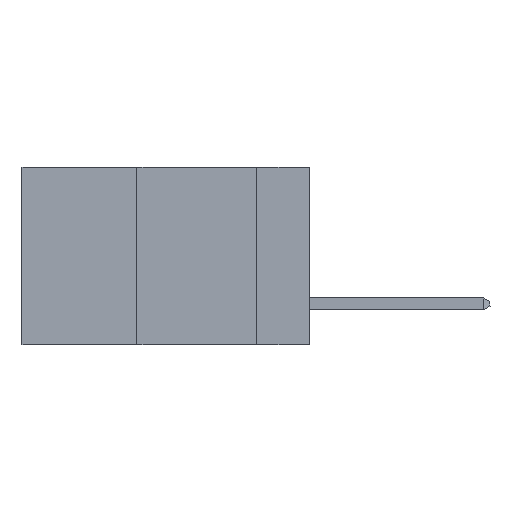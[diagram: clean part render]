
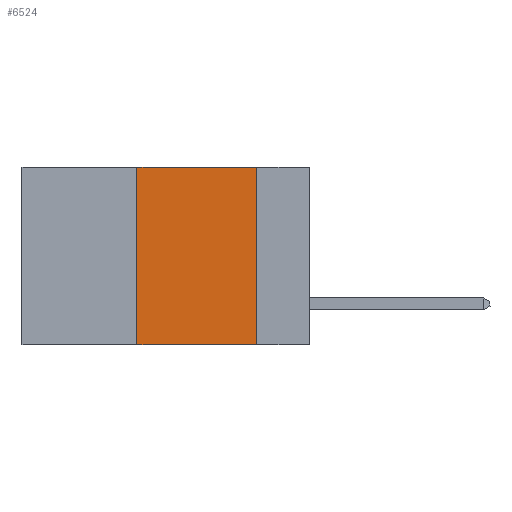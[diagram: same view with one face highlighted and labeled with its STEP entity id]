
A CAD part, left-side view. The second image highlights one B-rep face of the part: STEP entity #6524.
In plain terms, the highlighted planar face has unit normal (-1, 0, 0).
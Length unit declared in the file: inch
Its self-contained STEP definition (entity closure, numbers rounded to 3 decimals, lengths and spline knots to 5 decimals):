
#361 = DIRECTION ( 'NONE',  ( 0., -1., 0. ) ) ;
#2170 = EDGE_CURVE ( 'NONE', #18256, #9443, #5135, .T. ) ;
#4924 = CARTESIAN_POINT ( 'NONE',  ( 0., 0.11, -0.37 ) ) ;
#5135 = LINE ( 'NONE', #15441, #17207 ) ;
#6524 = ADVANCED_FACE ( 'NONE', ( #24255 ), #22433, .F. ) ;
#7306 = ORIENTED_EDGE ( 'NONE', *, *, #27800, .F. ) ;
#8111 = CARTESIAN_POINT ( 'NONE',  ( 0., 0.11, 0. ) ) ;
#8593 = LINE ( 'NONE', #22234, #20317 ) ;
#9443 = VERTEX_POINT ( 'NONE', #4924 ) ;
#10003 = ORIENTED_EDGE ( 'NONE', *, *, #2170, .F. ) ;
#10723 = CARTESIAN_POINT ( 'NONE',  ( 0., 0.36, 0. ) ) ;
#10781 = DIRECTION ( 'NONE',  ( 0., 0., 1. ) ) ;
#11017 = DIRECTION ( 'NONE',  ( 1., 0., 0. ) ) ;
#12390 = CARTESIAN_POINT ( 'NONE',  ( 0., 0.6, -0.37 ) ) ;
#13076 = VECTOR ( 'NONE', #26340, 39.37008 ) ;
#13789 = LINE ( 'NONE', #24116, #13076 ) ;
#14117 = LINE ( 'NONE', #12390, #26760 ) ;
#15441 = CARTESIAN_POINT ( 'NONE',  ( 0., 0.11, 0. ) ) ;
#17207 = VECTOR ( 'NONE', #19643, 39.37008 ) ;
#17431 = VERTEX_POINT ( 'NONE', #10723 ) ;
#17681 = EDGE_LOOP ( 'NONE', ( #10003, #7306, #18488, #19192 ) ) ;
#18256 = VERTEX_POINT ( 'NONE', #8111 ) ;
#18488 = ORIENTED_EDGE ( 'NONE', *, *, #27056, .F. ) ;
#19192 = ORIENTED_EDGE ( 'NONE', *, *, #28533, .T. ) ;
#19643 = DIRECTION ( 'NONE',  ( 0., 0., -1. ) ) ;
#20091 = AXIS2_PLACEMENT_3D ( 'NONE', #24651, #11017, #26853 ) ;
#20317 = VECTOR ( 'NONE', #10781, 39.37008 ) ;
#22234 = CARTESIAN_POINT ( 'NONE',  ( 0., 0.36, 0. ) ) ;
#22433 = PLANE ( 'NONE',  #20091 ) ;
#23125 = VERTEX_POINT ( 'NONE', #29838 ) ;
#24116 = CARTESIAN_POINT ( 'NONE',  ( 0., 0.6, 0. ) ) ;
#24255 = FACE_OUTER_BOUND ( 'NONE', #17681, .T. ) ;
#24651 = CARTESIAN_POINT ( 'NONE',  ( 0., 0.6, 0. ) ) ;
#26340 = DIRECTION ( 'NONE',  ( 0., -1., 0. ) ) ;
#26760 = VECTOR ( 'NONE', #361, 39.37008 ) ;
#26853 = DIRECTION ( 'NONE',  ( 0., 0., -1. ) ) ;
#27056 = EDGE_CURVE ( 'NONE', #23125, #17431, #8593, .T. ) ;
#27800 = EDGE_CURVE ( 'NONE', #17431, #18256, #13789, .T. ) ;
#28533 = EDGE_CURVE ( 'NONE', #23125, #9443, #14117, .T. ) ;
#29838 = CARTESIAN_POINT ( 'NONE',  ( 0., 0.36, -0.37 ) ) ;
